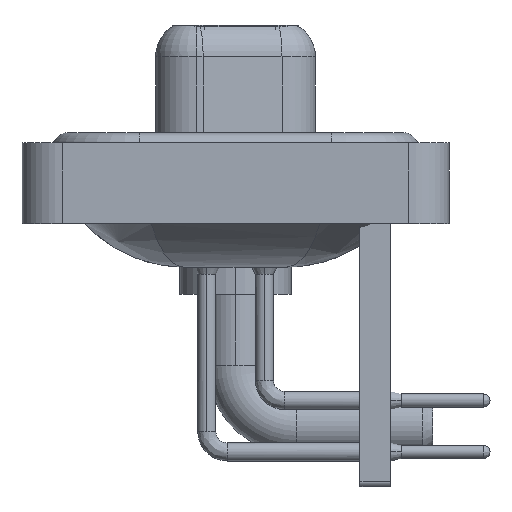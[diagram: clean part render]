
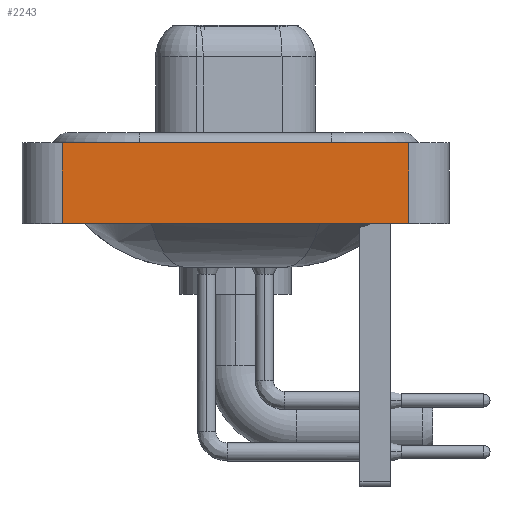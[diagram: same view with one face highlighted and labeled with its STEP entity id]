
A CAD part, left-side view. The second image highlights one B-rep face of the part: STEP entity #2243.
In plain terms, the highlighted planar face has unit normal (-1, 0, 0).
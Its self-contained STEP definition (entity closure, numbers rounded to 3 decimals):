
#633 = DIRECTION ( 'NONE',  ( 0., 0., 1. ) ) ;
#1252 = LINE ( 'NONE', #14522, #22840 ) ;
#1274 = ORIENTED_EDGE ( 'NONE', *, *, #6020, .F. ) ;
#2243 = ADVANCED_FACE ( 'NONE', ( #15575 ), #15462, .T. ) ;
#3227 = CARTESIAN_POINT ( 'NONE',  ( -7.3, 8.55, -3.6 ) ) ;
#5126 = DIRECTION ( 'NONE',  ( -1., 0., 0. ) ) ;
#5427 = EDGE_LOOP ( 'NONE', ( #11466, #1274, #11034, #9088 ) ) ;
#5459 = DIRECTION ( 'NONE',  ( 0., 0., 1. ) ) ;
#6020 = EDGE_CURVE ( 'NONE', #15203, #17444, #11751, .T. ) ;
#6446 = DIRECTION ( 'NONE',  ( 0., -1., 0. ) ) ;
#6527 = EDGE_CURVE ( 'NONE', #19217, #17444, #1252, .T. ) ;
#6604 = VECTOR ( 'NONE', #20155, 1000. ) ;
#9088 = ORIENTED_EDGE ( 'NONE', *, *, #18728, .T. ) ;
#9458 = CARTESIAN_POINT ( 'NONE',  ( -7.3, -8.55, -3.6 ) ) ;
#9750 = CARTESIAN_POINT ( 'NONE',  ( -7.3, -8.55, -3.6 ) ) ;
#9802 = CARTESIAN_POINT ( 'NONE',  ( -7.3, 8.55, -3.6 ) ) ;
#11034 = ORIENTED_EDGE ( 'NONE', *, *, #13170, .F. ) ;
#11453 = LINE ( 'NONE', #9802, #20568 ) ;
#11466 = ORIENTED_EDGE ( 'NONE', *, *, #6527, .T. ) ;
#11751 = LINE ( 'NONE', #19149, #16961 ) ;
#12846 = CARTESIAN_POINT ( 'NONE',  ( -7.3, -8.55, 0.4 ) ) ;
#13170 = EDGE_CURVE ( 'NONE', #20424, #15203, #11453, .T. ) ;
#13816 = CARTESIAN_POINT ( 'NONE',  ( -7.3, -8.55, -3.6 ) ) ;
#14522 = CARTESIAN_POINT ( 'NONE',  ( -7.3, -8.55, -3.6 ) ) ;
#15203 = VERTEX_POINT ( 'NONE', #19982 ) ;
#15462 = PLANE ( 'NONE',  #19466 ) ;
#15575 = FACE_OUTER_BOUND ( 'NONE', #5427, .T. ) ;
#16961 = VECTOR ( 'NONE', #6446, 1000. ) ;
#17444 = VERTEX_POINT ( 'NONE', #12846 ) ;
#18138 = DIRECTION ( 'NONE',  ( 0., 0., 1. ) ) ;
#18728 = EDGE_CURVE ( 'NONE', #20424, #19217, #21671, .T. ) ;
#19149 = CARTESIAN_POINT ( 'NONE',  ( -7.3, -8.55, 0.4 ) ) ;
#19217 = VERTEX_POINT ( 'NONE', #9750 ) ;
#19466 = AXIS2_PLACEMENT_3D ( 'NONE', #13816, #5126, #5459 ) ;
#19982 = CARTESIAN_POINT ( 'NONE',  ( -7.3, 8.55, 0.4 ) ) ;
#20155 = DIRECTION ( 'NONE',  ( 0., -1., 0. ) ) ;
#20424 = VERTEX_POINT ( 'NONE', #3227 ) ;
#20568 = VECTOR ( 'NONE', #633, 1000. ) ;
#21671 = LINE ( 'NONE', #9458, #6604 ) ;
#22840 = VECTOR ( 'NONE', #18138, 1000. ) ;
